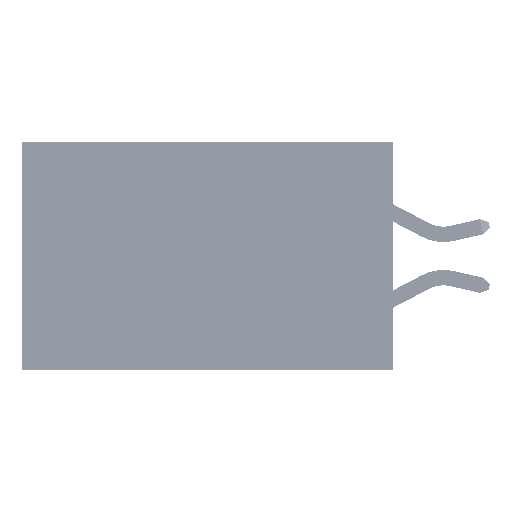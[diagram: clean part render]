
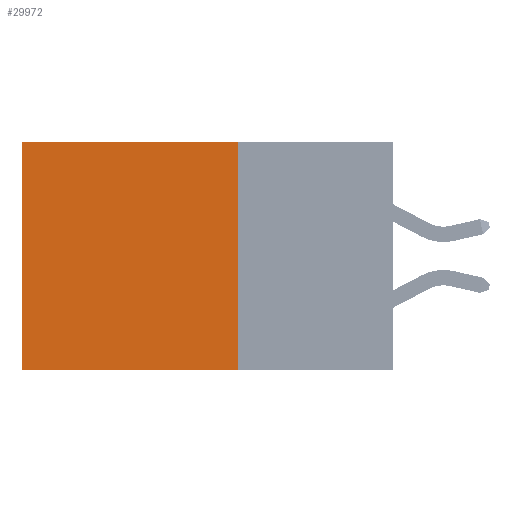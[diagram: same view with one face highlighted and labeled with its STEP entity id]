
A CAD part, left-side view. The second image highlights one B-rep face of the part: STEP entity #29972.
In plain terms, the highlighted planar face has unit normal (-1, 0, 0).
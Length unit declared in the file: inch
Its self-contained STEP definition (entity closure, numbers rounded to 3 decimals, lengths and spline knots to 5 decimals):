
#1825 = VERTEX_POINT ( 'NONE', #24932 ) ;
#3013 = VERTEX_POINT ( 'NONE', #24927 ) ;
#5186 = DIRECTION ( 'NONE',  ( 0., 0., -1. ) ) ;
#5285 = CARTESIAN_POINT ( 'NONE',  ( 0.2875, 0.25, -0.37 ) ) ;
#5504 = PLANE ( 'NONE',  #48168 ) ;
#6663 = FACE_OUTER_BOUND ( 'NONE', #41052, .T. ) ;
#7662 = LINE ( 'NONE', #5285, #18872 ) ;
#10042 = ORIENTED_EDGE ( 'NONE', *, *, #27710, .F. ) ;
#10715 = CARTESIAN_POINT ( 'NONE',  ( 0.2875, 0.6, 0. ) ) ;
#11467 = CARTESIAN_POINT ( 'NONE',  ( 0.2875, 0.6, -0.37 ) ) ;
#11494 = CARTESIAN_POINT ( 'NONE',  ( 0.2875, 0.25, 0. ) ) ;
#12158 = DIRECTION ( 'NONE',  ( 0., 1., 0. ) ) ;
#15439 = ORIENTED_EDGE ( 'NONE', *, *, #17791, .T. ) ;
#15457 = CARTESIAN_POINT ( 'NONE',  ( 0.2875, 0.25, 0. ) ) ;
#17791 = EDGE_CURVE ( 'NONE', #1825, #21673, #46882, .T. ) ;
#18872 = VECTOR ( 'NONE', #42985, 39.37008 ) ;
#20213 = VECTOR ( 'NONE', #12158, 39.37008 ) ;
#21614 = VECTOR ( 'NONE', #40504, 39.37008 ) ;
#21673 = VERTEX_POINT ( 'NONE', #11467 ) ;
#22716 = ORIENTED_EDGE ( 'NONE', *, *, #38310, .T. ) ;
#24927 = CARTESIAN_POINT ( 'NONE',  ( 0.2875, 0.25, -0.37 ) ) ;
#24932 = CARTESIAN_POINT ( 'NONE',  ( 0.2875, 0.6, 0. ) ) ;
#27710 = EDGE_CURVE ( 'NONE', #29642, #3013, #28700, .T. ) ;
#28253 = DIRECTION ( 'NONE',  ( 1., 0., 0. ) ) ;
#28700 = LINE ( 'NONE', #46508, #45794 ) ;
#28891 = ORIENTED_EDGE ( 'NONE', *, *, #45364, .F. ) ;
#29642 = VERTEX_POINT ( 'NONE', #11494 ) ;
#29972 = ADVANCED_FACE ( 'NONE', ( #6663 ), #5504, .F. ) ;
#31864 = CARTESIAN_POINT ( 'NONE',  ( 0.2875, 0.25, 0. ) ) ;
#35821 = DIRECTION ( 'NONE',  ( 0., 0., -1. ) ) ;
#37255 = LINE ( 'NONE', #15457, #20213 ) ;
#38310 = EDGE_CURVE ( 'NONE', #29642, #1825, #37255, .T. ) ;
#40504 = DIRECTION ( 'NONE',  ( 0., 0., -1. ) ) ;
#41052 = EDGE_LOOP ( 'NONE', ( #15439, #28891, #10042, #22716 ) ) ;
#42985 = DIRECTION ( 'NONE',  ( 0., 1., 0. ) ) ;
#45364 = EDGE_CURVE ( 'NONE', #3013, #21673, #7662, .T. ) ;
#45794 = VECTOR ( 'NONE', #5186, 39.37008 ) ;
#46508 = CARTESIAN_POINT ( 'NONE',  ( 0.2875, 0.25, 0. ) ) ;
#46882 = LINE ( 'NONE', #10715, #21614 ) ;
#48168 = AXIS2_PLACEMENT_3D ( 'NONE', #31864, #28253, #35821 ) ;
